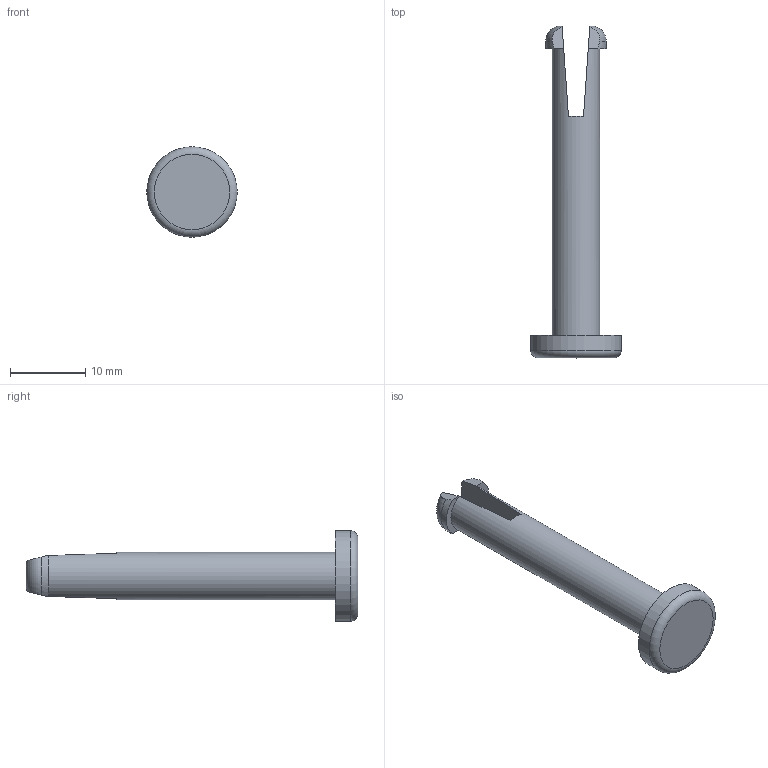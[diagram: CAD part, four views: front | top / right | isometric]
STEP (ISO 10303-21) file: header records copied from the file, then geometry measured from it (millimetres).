
FILE_DESCRIPTION(/* description */ (''),/* implementation_level */ '2;1');
FILE_NAME(/* name */ 'Rear_Snap_Pin.stp',/* time_stamp */ '2015-01-06T20:43:13-06:00',/* author */ (''),/* organization */ (''),/* preprocessor_version */ 'ST-DEVELOPER v14.6',/* originating_system */ '',/* authorisation */ '');
FILE_SCHEMA (('AUTOMOTIVE_DESIGN { 1 2 10303 214 1 1 1 1 }'));
Length unit declared in the file: centimetre
Products named in the file (1): 1234-K789
Bounding box: 12 x 44 x 12 mm (x, y, z)
Volume: 1421.7 mm3; surface area: 1203.2 mm2
Topology: 1 solids, 1 shells, 22 faces, 56 edges, 37 vertices
Faces by surface type: plane 15, cylinder 4, torus 3
Full cylindrical faces by diameter (mm): 6.3 x1, 12 x1
Entity records: 1171 total; most frequent: CARTESIAN_POINT 627, DIRECTION 114, ORIENTED_EDGE 104, EDGE_CURVE 52, AXIS2_PLACEMENT_3D 47, VERTEX_POINT 36, EDGE_LOOP 26, FACE_OUTER_BOUND 22
